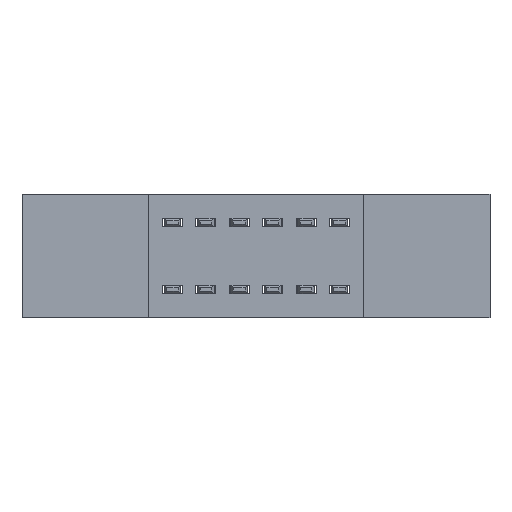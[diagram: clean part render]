
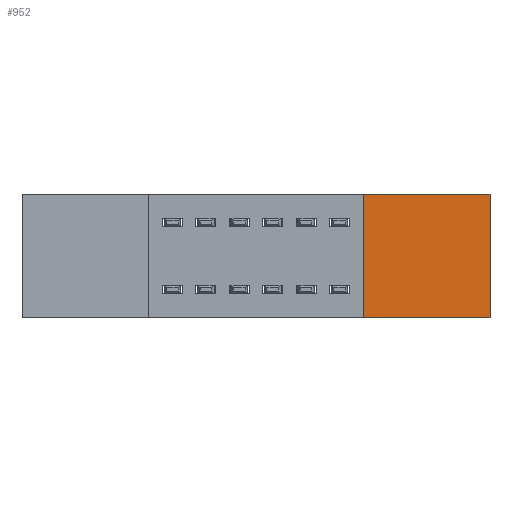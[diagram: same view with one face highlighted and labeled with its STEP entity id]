
A CAD part, front view. The second image highlights one B-rep face of the part: STEP entity #952.
In plain terms, the highlighted planar face has unit normal (0, -1, 0).
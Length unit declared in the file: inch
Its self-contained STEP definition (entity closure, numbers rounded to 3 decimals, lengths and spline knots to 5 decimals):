
#59 = CARTESIAN_POINT ( 'NONE',  ( 1.023, 0., 0. ) ) ;
#240 = CARTESIAN_POINT ( 'NONE',  ( 0., 0., 0. ) ) ;
#451 = FACE_OUTER_BOUND ( 'NONE', #1460, .T. ) ;
#630 = VERTEX_POINT ( 'NONE', #5542 ) ;
#795 = CARTESIAN_POINT ( 'NONE',  ( 0., 0., -0.37 ) ) ;
#952 = ADVANCED_FACE ( 'NONE', ( #451 ), #2808, .T. ) ;
#1460 = EDGE_LOOP ( 'NONE', ( #3292, #5106, #2113, #7914 ) ) ;
#1751 = VECTOR ( 'NONE', #6017, 39.37008 ) ;
#2113 = ORIENTED_EDGE ( 'NONE', *, *, #7135, .F. ) ;
#2254 = VECTOR ( 'NONE', #3002, 39.37008 ) ;
#2489 = EDGE_CURVE ( 'NONE', #7592, #630, #4134, .T. ) ;
#2710 = VECTOR ( 'NONE', #5645, 39.37008 ) ;
#2773 = CARTESIAN_POINT ( 'NONE',  ( 0., 0., -0.37 ) ) ;
#2808 = PLANE ( 'NONE',  #4423 ) ;
#2887 = VERTEX_POINT ( 'NONE', #8090 ) ;
#2957 = EDGE_CURVE ( 'NONE', #2887, #5317, #5051, .T. ) ;
#3002 = DIRECTION ( 'NONE',  ( 1., 0., 0. ) ) ;
#3292 = ORIENTED_EDGE ( 'NONE', *, *, #4554, .F. ) ;
#3413 = LINE ( 'NONE', #5547, #1751 ) ;
#4134 = LINE ( 'NONE', #240, #2254 ) ;
#4423 = AXIS2_PLACEMENT_3D ( 'NONE', #795, #4472, #4926 ) ;
#4472 = DIRECTION ( 'NONE',  ( 0., -1., 0. ) ) ;
#4501 = CARTESIAN_POINT ( 'NONE',  ( 1.023, 0., -0.37 ) ) ;
#4554 = EDGE_CURVE ( 'NONE', #5317, #7592, #5738, .T. ) ;
#4926 = DIRECTION ( 'NONE',  ( 0., 0., -1. ) ) ;
#5051 = LINE ( 'NONE', #2773, #6976 ) ;
#5106 = ORIENTED_EDGE ( 'NONE', *, *, #2957, .F. ) ;
#5317 = VERTEX_POINT ( 'NONE', #4501 ) ;
#5542 = CARTESIAN_POINT ( 'NONE',  ( 1.4, 0., 0. ) ) ;
#5547 = CARTESIAN_POINT ( 'NONE',  ( 1.4, 0., 0. ) ) ;
#5645 = DIRECTION ( 'NONE',  ( 0., 0., 1. ) ) ;
#5738 = LINE ( 'NONE', #7595, #2710 ) ;
#6017 = DIRECTION ( 'NONE',  ( 0., 0., -1. ) ) ;
#6976 = VECTOR ( 'NONE', #7108, 39.37008 ) ;
#7108 = DIRECTION ( 'NONE',  ( -1., 0., 0. ) ) ;
#7135 = EDGE_CURVE ( 'NONE', #630, #2887, #3413, .T. ) ;
#7592 = VERTEX_POINT ( 'NONE', #59 ) ;
#7595 = CARTESIAN_POINT ( 'NONE',  ( 1.023, 0., -0.37 ) ) ;
#7914 = ORIENTED_EDGE ( 'NONE', *, *, #2489, .F. ) ;
#8090 = CARTESIAN_POINT ( 'NONE',  ( 1.4, 0., -0.37 ) ) ;
